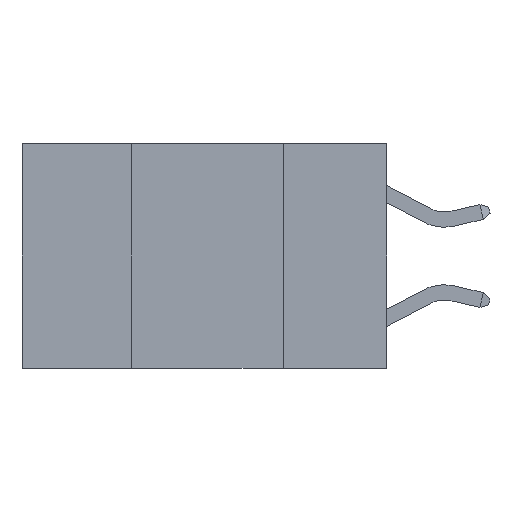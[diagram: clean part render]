
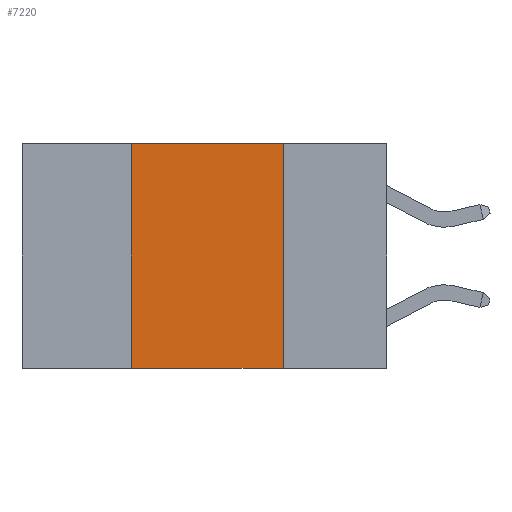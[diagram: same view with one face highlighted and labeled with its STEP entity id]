
A CAD part, left-side view. The second image highlights one B-rep face of the part: STEP entity #7220.
In plain terms, the highlighted planar face has unit normal (-1, 0, 0).
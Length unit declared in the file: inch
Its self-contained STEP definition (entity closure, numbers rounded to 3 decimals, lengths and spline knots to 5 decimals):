
#635 = ORIENTED_EDGE ( 'NONE', *, *, #6546, .F. ) ;
#690 = VERTEX_POINT ( 'NONE', #2429 ) ;
#859 = LINE ( 'NONE', #4536, #2981 ) ;
#1161 = VECTOR ( 'NONE', #9418, 39.37008 ) ;
#1451 = VECTOR ( 'NONE', #6430, 39.37008 ) ;
#1550 = VERTEX_POINT ( 'NONE', #9023 ) ;
#2429 = CARTESIAN_POINT ( 'NONE',  ( 0., 0.42, 0. ) ) ;
#2663 = VERTEX_POINT ( 'NONE', #4492 ) ;
#2819 = ORIENTED_EDGE ( 'NONE', *, *, #6025, .F. ) ;
#2981 = VECTOR ( 'NONE', #9005, 39.37008 ) ;
#3097 = FACE_OUTER_BOUND ( 'NONE', #9726, .T. ) ;
#3735 = CARTESIAN_POINT ( 'NONE',  ( 0., 0.6, 0. ) ) ;
#4492 = CARTESIAN_POINT ( 'NONE',  ( 0., 0.17, -0.37 ) ) ;
#4536 = CARTESIAN_POINT ( 'NONE',  ( 0., 0.17, 0. ) ) ;
#4979 = VECTOR ( 'NONE', #5529, 39.37008 ) ;
#5136 = EDGE_CURVE ( 'NONE', #690, #11393, #6281, .T. ) ;
#5529 = DIRECTION ( 'NONE',  ( 0., -1., 0. ) ) ;
#5531 = DIRECTION ( 'NONE',  ( 0., 0., -1. ) ) ;
#5961 = LINE ( 'NONE', #6714, #1161 ) ;
#6025 = EDGE_CURVE ( 'NONE', #1550, #690, #5961, .T. ) ;
#6281 = LINE ( 'NONE', #9997, #1451 ) ;
#6430 = DIRECTION ( 'NONE',  ( 0., -1., 0. ) ) ;
#6446 = CARTESIAN_POINT ( 'NONE',  ( 0., 0.6, -0.37 ) ) ;
#6546 = EDGE_CURVE ( 'NONE', #11393, #2663, #859, .T. ) ;
#6714 = CARTESIAN_POINT ( 'NONE',  ( 0., 0.42, 0. ) ) ;
#7220 = ADVANCED_FACE ( 'NONE', ( #3097 ), #9101, .F. ) ;
#7391 = LINE ( 'NONE', #6446, #4979 ) ;
#8646 = ORIENTED_EDGE ( 'NONE', *, *, #5136, .F. ) ;
#8669 = CARTESIAN_POINT ( 'NONE',  ( 0., 0.17, 0. ) ) ;
#9005 = DIRECTION ( 'NONE',  ( 0., 0., -1. ) ) ;
#9023 = CARTESIAN_POINT ( 'NONE',  ( 0., 0.42, -0.37 ) ) ;
#9101 = PLANE ( 'NONE',  #10012 ) ;
#9418 = DIRECTION ( 'NONE',  ( 0., 0., 1. ) ) ;
#9726 = EDGE_LOOP ( 'NONE', ( #635, #8646, #2819, #10086 ) ) ;
#9997 = CARTESIAN_POINT ( 'NONE',  ( 0., 0.6, 0. ) ) ;
#10012 = AXIS2_PLACEMENT_3D ( 'NONE', #3735, #10958, #5531 ) ;
#10086 = ORIENTED_EDGE ( 'NONE', *, *, #11112, .T. ) ;
#10958 = DIRECTION ( 'NONE',  ( 1., 0., 0. ) ) ;
#11112 = EDGE_CURVE ( 'NONE', #1550, #2663, #7391, .T. ) ;
#11393 = VERTEX_POINT ( 'NONE', #8669 ) ;
